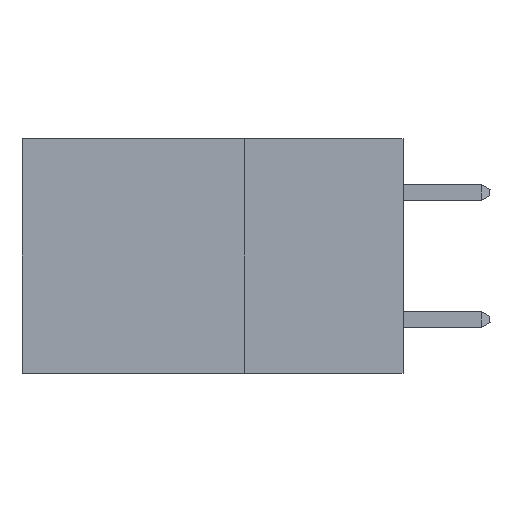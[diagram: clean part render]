
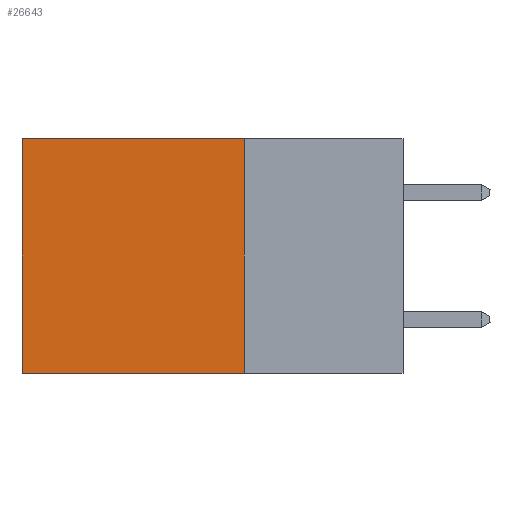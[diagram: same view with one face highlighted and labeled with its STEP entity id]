
A CAD part, left-side view. The second image highlights one B-rep face of the part: STEP entity #26643.
In plain terms, the highlighted planar face has unit normal (-1, 0, 0).
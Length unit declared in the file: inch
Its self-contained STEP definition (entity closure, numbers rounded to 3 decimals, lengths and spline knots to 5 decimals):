
#1067 = DIRECTION ( 'NONE',  ( 0., 1., 0. ) ) ;
#2250 = CARTESIAN_POINT ( 'NONE',  ( 0.2875, 0.6, 0. ) ) ;
#2319 = CARTESIAN_POINT ( 'NONE',  ( 0.2875, 0.25, -0.37 ) ) ;
#3032 = CARTESIAN_POINT ( 'NONE',  ( 0.2875, 0.6, 0. ) ) ;
#3306 = CARTESIAN_POINT ( 'NONE',  ( 0.2875, 0.25, 0. ) ) ;
#3463 = LINE ( 'NONE', #3032, #10644 ) ;
#4235 = LINE ( 'NONE', #2319, #14365 ) ;
#7331 = DIRECTION ( 'NONE',  ( 1., 0., 0. ) ) ;
#7830 = ORIENTED_EDGE ( 'NONE', *, *, #25927, .T. ) ;
#9426 = ORIENTED_EDGE ( 'NONE', *, *, #15976, .F. ) ;
#10644 = VECTOR ( 'NONE', #17918, 39.37008 ) ;
#11018 = VERTEX_POINT ( 'NONE', #23965 ) ;
#11241 = EDGE_CURVE ( 'NONE', #21113, #17996, #4235, .T. ) ;
#12101 = CARTESIAN_POINT ( 'NONE',  ( 0.2875, 0.6, -0.37 ) ) ;
#12508 = CARTESIAN_POINT ( 'NONE',  ( 0.2875, 0.25, -0.37 ) ) ;
#13902 = PLANE ( 'NONE',  #17052 ) ;
#14005 = EDGE_CURVE ( 'NONE', #25722, #17996, #3463, .T. ) ;
#14288 = LINE ( 'NONE', #25700, #19163 ) ;
#14365 = VECTOR ( 'NONE', #25419, 39.37008 ) ;
#15389 = EDGE_LOOP ( 'NONE', ( #24425, #20117, #9426, #7830 ) ) ;
#15976 = EDGE_CURVE ( 'NONE', #11018, #21113, #14288, .T. ) ;
#17052 = AXIS2_PLACEMENT_3D ( 'NONE', #3306, #7331, #23934 ) ;
#17534 = LINE ( 'NONE', #24151, #18847 ) ;
#17918 = DIRECTION ( 'NONE',  ( 0., 0., -1. ) ) ;
#17996 = VERTEX_POINT ( 'NONE', #12101 ) ;
#18847 = VECTOR ( 'NONE', #1067, 39.37008 ) ;
#19163 = VECTOR ( 'NONE', #26068, 39.37008 ) ;
#20117 = ORIENTED_EDGE ( 'NONE', *, *, #11241, .F. ) ;
#21113 = VERTEX_POINT ( 'NONE', #12508 ) ;
#21717 = FACE_OUTER_BOUND ( 'NONE', #15389, .T. ) ;
#23934 = DIRECTION ( 'NONE',  ( 0., 0., -1. ) ) ;
#23965 = CARTESIAN_POINT ( 'NONE',  ( 0.2875, 0.25, 0. ) ) ;
#24151 = CARTESIAN_POINT ( 'NONE',  ( 0.2875, 0.25, 0. ) ) ;
#24425 = ORIENTED_EDGE ( 'NONE', *, *, #14005, .T. ) ;
#25419 = DIRECTION ( 'NONE',  ( 0., 1., 0. ) ) ;
#25700 = CARTESIAN_POINT ( 'NONE',  ( 0.2875, 0.25, 0. ) ) ;
#25722 = VERTEX_POINT ( 'NONE', #2250 ) ;
#25927 = EDGE_CURVE ( 'NONE', #11018, #25722, #17534, .T. ) ;
#26068 = DIRECTION ( 'NONE',  ( 0., 0., -1. ) ) ;
#26643 = ADVANCED_FACE ( 'NONE', ( #21717 ), #13902, .F. ) ;
